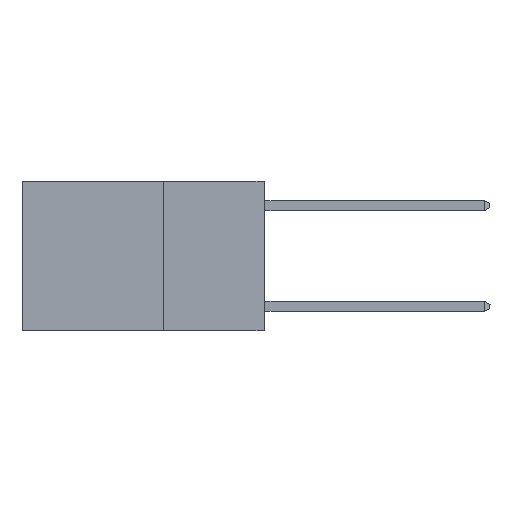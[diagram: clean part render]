
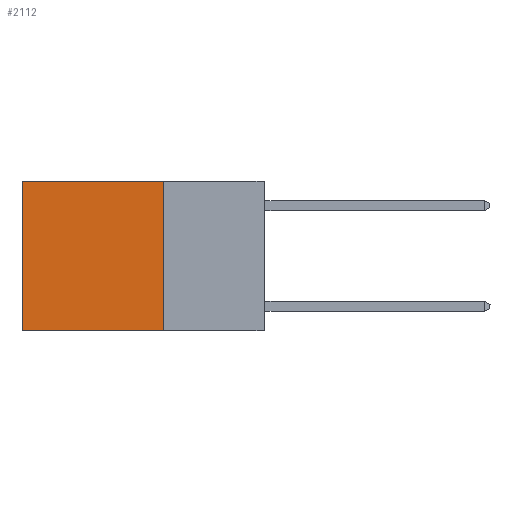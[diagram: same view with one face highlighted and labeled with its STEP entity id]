
A CAD part, left-side view. The second image highlights one B-rep face of the part: STEP entity #2112.
In plain terms, the highlighted planar face has unit normal (-1, 0, 0).
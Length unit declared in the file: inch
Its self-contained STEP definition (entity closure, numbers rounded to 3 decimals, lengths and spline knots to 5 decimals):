
#1935 = VERTEX_POINT ( 'NONE', #11453 ) ;
#2112 = ADVANCED_FACE ( 'NONE', ( #12730 ), #5148, .F. ) ;
#2255 = VECTOR ( 'NONE', #7697, 39.37008 ) ;
#2825 = CARTESIAN_POINT ( 'NONE',  ( 0.2625, 0.6, -0.37 ) ) ;
#3702 = AXIS2_PLACEMENT_3D ( 'NONE', #12972, #14046, #7403 ) ;
#3704 = ORIENTED_EDGE ( 'NONE', *, *, #11145, .F. ) ;
#4142 = VECTOR ( 'NONE', #6648, 39.37008 ) ;
#4723 = EDGE_CURVE ( 'NONE', #5109, #1935, #9153, .T. ) ;
#4770 = ORIENTED_EDGE ( 'NONE', *, *, #6348, .T. ) ;
#5054 = CARTESIAN_POINT ( 'NONE',  ( 0.2625, 0.6, 0. ) ) ;
#5109 = VERTEX_POINT ( 'NONE', #12550 ) ;
#5148 = PLANE ( 'NONE',  #3702 ) ;
#5282 = ORIENTED_EDGE ( 'NONE', *, *, #10894, .T. ) ;
#5430 = VECTOR ( 'NONE', #6192, 39.37008 ) ;
#5597 = LINE ( 'NONE', #14340, #2255 ) ;
#5982 = VERTEX_POINT ( 'NONE', #13843 ) ;
#6192 = DIRECTION ( 'NONE',  ( 0., 0., -1. ) ) ;
#6200 = VECTOR ( 'NONE', #10789, 39.37008 ) ;
#6348 = EDGE_CURVE ( 'NONE', #5109, #5982, #7493, .T. ) ;
#6648 = DIRECTION ( 'NONE',  ( 0., 1., 0. ) ) ;
#7403 = DIRECTION ( 'NONE',  ( 0., 0., -1. ) ) ;
#7493 = LINE ( 'NONE', #13326, #4142 ) ;
#7697 = DIRECTION ( 'NONE',  ( 0., 1., 0. ) ) ;
#8274 = EDGE_LOOP ( 'NONE', ( #5282, #3704, #13329, #4770 ) ) ;
#8546 = CARTESIAN_POINT ( 'NONE',  ( 0.2625, 0.25, 0. ) ) ;
#9153 = LINE ( 'NONE', #8546, #6200 ) ;
#9451 = LINE ( 'NONE', #5054, #5430 ) ;
#10789 = DIRECTION ( 'NONE',  ( 0., 0., -1. ) ) ;
#10894 = EDGE_CURVE ( 'NONE', #5982, #13996, #9451, .T. ) ;
#11145 = EDGE_CURVE ( 'NONE', #1935, #13996, #5597, .T. ) ;
#11453 = CARTESIAN_POINT ( 'NONE',  ( 0.2625, 0.25, -0.37 ) ) ;
#12550 = CARTESIAN_POINT ( 'NONE',  ( 0.2625, 0.25, 0. ) ) ;
#12730 = FACE_OUTER_BOUND ( 'NONE', #8274, .T. ) ;
#12972 = CARTESIAN_POINT ( 'NONE',  ( 0.2625, 0.25, 0. ) ) ;
#13326 = CARTESIAN_POINT ( 'NONE',  ( 0.2625, 0.25, 0. ) ) ;
#13329 = ORIENTED_EDGE ( 'NONE', *, *, #4723, .F. ) ;
#13843 = CARTESIAN_POINT ( 'NONE',  ( 0.2625, 0.6, 0. ) ) ;
#13996 = VERTEX_POINT ( 'NONE', #2825 ) ;
#14046 = DIRECTION ( 'NONE',  ( 1., 0., 0. ) ) ;
#14340 = CARTESIAN_POINT ( 'NONE',  ( 0.2625, 0.25, -0.37 ) ) ;
